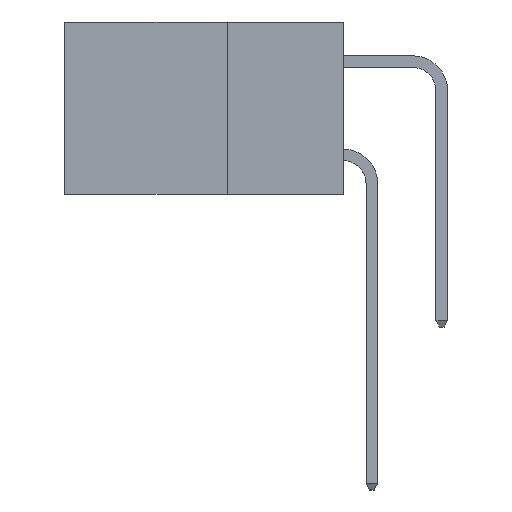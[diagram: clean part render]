
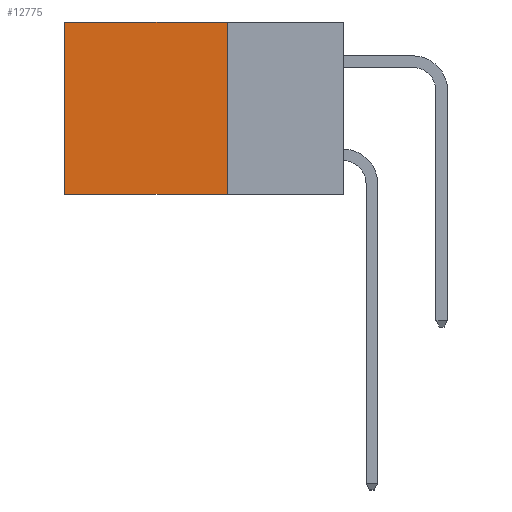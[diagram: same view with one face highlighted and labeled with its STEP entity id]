
A CAD part, left-side view. The second image highlights one B-rep face of the part: STEP entity #12775.
In plain terms, the highlighted planar face has unit normal (-1, 0, 0).
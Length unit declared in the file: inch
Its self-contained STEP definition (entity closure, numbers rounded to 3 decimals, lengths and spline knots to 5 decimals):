
#539 = ORIENTED_EDGE ( 'NONE', *, *, #2135, .F. ) ;
#662 = DIRECTION ( 'NONE',  ( 1., 0., 0. ) ) ;
#668 = DIRECTION ( 'NONE',  ( 0., 0., -1. ) ) ;
#892 = CARTESIAN_POINT ( 'NONE',  ( 0.2615, 0.6, -0.37 ) ) ;
#1066 = LINE ( 'NONE', #13456, #3786 ) ;
#1547 = EDGE_CURVE ( 'NONE', #10310, #8887, #9419, .T. ) ;
#1828 = PLANE ( 'NONE',  #13431 ) ;
#2135 = EDGE_CURVE ( 'NONE', #10310, #4887, #4494, .T. ) ;
#2649 = LINE ( 'NONE', #5562, #8082 ) ;
#3264 = ORIENTED_EDGE ( 'NONE', *, *, #1547, .T. ) ;
#3309 = CARTESIAN_POINT ( 'NONE',  ( 0.2615, 0.25, 0. ) ) ;
#3419 = CARTESIAN_POINT ( 'NONE',  ( 0.2615, 0.25, -0.37 ) ) ;
#3698 = EDGE_LOOP ( 'NONE', ( #7551, #6658, #539, #3264 ) ) ;
#3786 = VECTOR ( 'NONE', #7671, 39.37008 ) ;
#4036 = DIRECTION ( 'NONE',  ( 0., 1., 0. ) ) ;
#4494 = LINE ( 'NONE', #3419, #7587 ) ;
#4887 = VERTEX_POINT ( 'NONE', #9931 ) ;
#5233 = FACE_OUTER_BOUND ( 'NONE', #3698, .T. ) ;
#5293 = DIRECTION ( 'NONE',  ( 0., 1., 0. ) ) ;
#5327 = CARTESIAN_POINT ( 'NONE',  ( 0.2615, 0.25, -0.37 ) ) ;
#5562 = CARTESIAN_POINT ( 'NONE',  ( 0.2615, 0.25, -0.37 ) ) ;
#6658 = ORIENTED_EDGE ( 'NONE', *, *, #7602, .F. ) ;
#7551 = ORIENTED_EDGE ( 'NONE', *, *, #11462, .T. ) ;
#7587 = VECTOR ( 'NONE', #668, 39.37008 ) ;
#7602 = EDGE_CURVE ( 'NONE', #4887, #8755, #2649, .T. ) ;
#7671 = DIRECTION ( 'NONE',  ( 0., 0., -1. ) ) ;
#8082 = VECTOR ( 'NONE', #5293, 39.37008 ) ;
#8755 = VERTEX_POINT ( 'NONE', #892 ) ;
#8829 = DIRECTION ( 'NONE',  ( 0., 0., -1. ) ) ;
#8887 = VERTEX_POINT ( 'NONE', #13899 ) ;
#9419 = LINE ( 'NONE', #3309, #12160 ) ;
#9670 = CARTESIAN_POINT ( 'NONE',  ( 0.2615, 0.25, 0. ) ) ;
#9931 = CARTESIAN_POINT ( 'NONE',  ( 0.2615, 0.25, -0.37 ) ) ;
#10310 = VERTEX_POINT ( 'NONE', #9670 ) ;
#11462 = EDGE_CURVE ( 'NONE', #8887, #8755, #1066, .T. ) ;
#12160 = VECTOR ( 'NONE', #4036, 39.37008 ) ;
#12775 = ADVANCED_FACE ( 'NONE', ( #5233 ), #1828, .F. ) ;
#13431 = AXIS2_PLACEMENT_3D ( 'NONE', #5327, #662, #8829 ) ;
#13456 = CARTESIAN_POINT ( 'NONE',  ( 0.2615, 0.6, -0.37 ) ) ;
#13899 = CARTESIAN_POINT ( 'NONE',  ( 0.2615, 0.6, 0. ) ) ;
